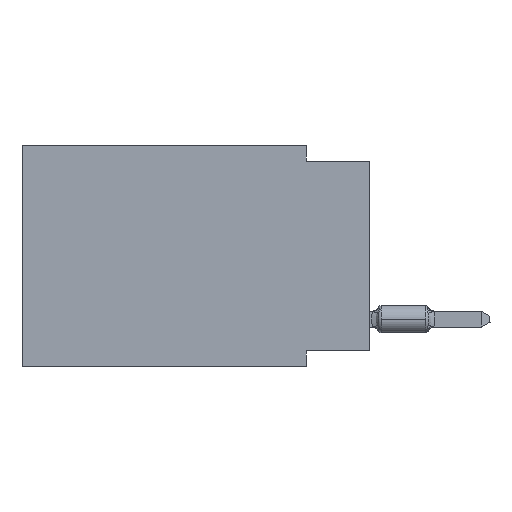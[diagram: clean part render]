
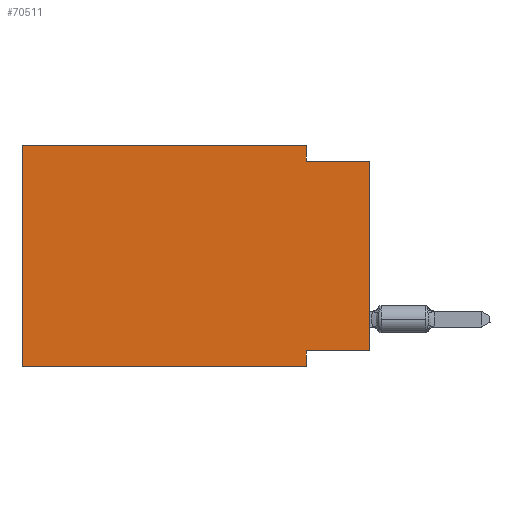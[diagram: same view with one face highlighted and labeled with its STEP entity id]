
A CAD part, left-side view. The second image highlights one B-rep face of the part: STEP entity #70511.
In plain terms, the highlighted planar face has unit normal (-1, 0, 0).
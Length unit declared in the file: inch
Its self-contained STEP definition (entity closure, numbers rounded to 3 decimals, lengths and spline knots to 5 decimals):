
#1598 = CARTESIAN_POINT ( 'NONE',  ( 0., 0.1, -0.35 ) ) ;
#3187 = DIRECTION ( 'NONE',  ( 0., -1., 0. ) ) ;
#3453 = EDGE_CURVE ( 'NONE', #14764, #11191, #44569, .T. ) ;
#3524 = CARTESIAN_POINT ( 'NONE',  ( 0., 0.55, 0. ) ) ;
#4413 = EDGE_LOOP ( 'NONE', ( #73870, #33996, #69466, #9578, #38629, #67744, #40566, #40984 ) ) ;
#5524 = CARTESIAN_POINT ( 'NONE',  ( 0., 0., -0.325 ) ) ;
#7587 = EDGE_CURVE ( 'NONE', #51662, #61968, #21313, .T. ) ;
#7696 = CARTESIAN_POINT ( 'NONE',  ( 0., 0.55, 0. ) ) ;
#7808 = LINE ( 'NONE', #31062, #12191 ) ;
#9064 = VECTOR ( 'NONE', #9589, 39.37008 ) ;
#9578 = ORIENTED_EDGE ( 'NONE', *, *, #29497, .F. ) ;
#9589 = DIRECTION ( 'NONE',  ( 0., 0., -1. ) ) ;
#10013 = LINE ( 'NONE', #51193, #49766 ) ;
#11093 = DIRECTION ( 'NONE',  ( 0., 0., 1. ) ) ;
#11191 = VERTEX_POINT ( 'NONE', #22065 ) ;
#12191 = VECTOR ( 'NONE', #25345, 39.37008 ) ;
#13941 = CARTESIAN_POINT ( 'NONE',  ( 0., 0.55, -0.35 ) ) ;
#14764 = VERTEX_POINT ( 'NONE', #15960 ) ;
#15960 = CARTESIAN_POINT ( 'NONE',  ( 0., 0.1, 0. ) ) ;
#19784 = CARTESIAN_POINT ( 'NONE',  ( 0., 0.1, 0. ) ) ;
#21313 = LINE ( 'NONE', #44572, #62025 ) ;
#22065 = CARTESIAN_POINT ( 'NONE',  ( 0., 0.1, -0.025 ) ) ;
#22476 = VECTOR ( 'NONE', #35885, 39.37008 ) ;
#25276 = VERTEX_POINT ( 'NONE', #5524 ) ;
#25345 = DIRECTION ( 'NONE',  ( 0., -1., 0. ) ) ;
#25896 = DIRECTION ( 'NONE',  ( 0., 0., -1. ) ) ;
#27191 = LINE ( 'NONE', #50457, #53890 ) ;
#28272 = VERTEX_POINT ( 'NONE', #1598 ) ;
#29497 = EDGE_CURVE ( 'NONE', #61968, #14764, #10013, .T. ) ;
#31062 = CARTESIAN_POINT ( 'NONE',  ( 0., 0.55, -0.35 ) ) ;
#33996 = ORIENTED_EDGE ( 'NONE', *, *, #38897, .F. ) ;
#34585 = VERTEX_POINT ( 'NONE', #64660 ) ;
#35885 = DIRECTION ( 'NONE',  ( 0., 1., 0. ) ) ;
#38629 = ORIENTED_EDGE ( 'NONE', *, *, #7587, .F. ) ;
#38897 = EDGE_CURVE ( 'NONE', #11191, #34585, #27191, .T. ) ;
#38972 = CARTESIAN_POINT ( 'NONE',  ( 0., 0., 0. ) ) ;
#39345 = PLANE ( 'NONE',  #42249 ) ;
#39721 = FACE_OUTER_BOUND ( 'NONE', #4413, .T. ) ;
#40566 = ORIENTED_EDGE ( 'NONE', *, *, #67589, .F. ) ;
#40984 = ORIENTED_EDGE ( 'NONE', *, *, #43044, .F. ) ;
#42249 = AXIS2_PLACEMENT_3D ( 'NONE', #3524, #50044, #74420 ) ;
#43044 = EDGE_CURVE ( 'NONE', #25276, #46125, #65608, .T. ) ;
#44336 = DIRECTION ( 'NONE',  ( 0., -1., 0. ) ) ;
#44569 = LINE ( 'NONE', #19784, #58536 ) ;
#44572 = CARTESIAN_POINT ( 'NONE',  ( 0., 0.55, 0. ) ) ;
#46125 = VERTEX_POINT ( 'NONE', #59678 ) ;
#47813 = VECTOR ( 'NONE', #11093, 39.37008 ) ;
#48064 = CARTESIAN_POINT ( 'NONE',  ( 0., 0., -0.325 ) ) ;
#49766 = VECTOR ( 'NONE', #44336, 39.37008 ) ;
#50044 = DIRECTION ( 'NONE',  ( 1., 0., 0. ) ) ;
#50457 = CARTESIAN_POINT ( 'NONE',  ( 0., 0., -0.025 ) ) ;
#51193 = CARTESIAN_POINT ( 'NONE',  ( 0., 0.55, 0. ) ) ;
#51662 = VERTEX_POINT ( 'NONE', #13941 ) ;
#53890 = VECTOR ( 'NONE', #3187, 39.37008 ) ;
#56131 = LINE ( 'NONE', #38972, #47813 ) ;
#57210 = EDGE_CURVE ( 'NONE', #51662, #28272, #7808, .T. ) ;
#58536 = VECTOR ( 'NONE', #25896, 39.37008 ) ;
#59678 = CARTESIAN_POINT ( 'NONE',  ( 0., 0.1, -0.325 ) ) ;
#61833 = CARTESIAN_POINT ( 'NONE',  ( 0., 0.1, -0.35 ) ) ;
#61968 = VERTEX_POINT ( 'NONE', #7696 ) ;
#62025 = VECTOR ( 'NONE', #67828, 39.37008 ) ;
#64156 = EDGE_CURVE ( 'NONE', #25276, #34585, #56131, .T. ) ;
#64660 = CARTESIAN_POINT ( 'NONE',  ( 0., 0., -0.025 ) ) ;
#65608 = LINE ( 'NONE', #48064, #22476 ) ;
#66417 = LINE ( 'NONE', #61833, #9064 ) ;
#67589 = EDGE_CURVE ( 'NONE', #46125, #28272, #66417, .T. ) ;
#67744 = ORIENTED_EDGE ( 'NONE', *, *, #57210, .T. ) ;
#67828 = DIRECTION ( 'NONE',  ( 0., 0., 1. ) ) ;
#69466 = ORIENTED_EDGE ( 'NONE', *, *, #3453, .F. ) ;
#70511 = ADVANCED_FACE ( 'NONE', ( #39721 ), #39345, .F. ) ;
#73870 = ORIENTED_EDGE ( 'NONE', *, *, #64156, .T. ) ;
#74420 = DIRECTION ( 'NONE',  ( 0., 0., -1. ) ) ;
